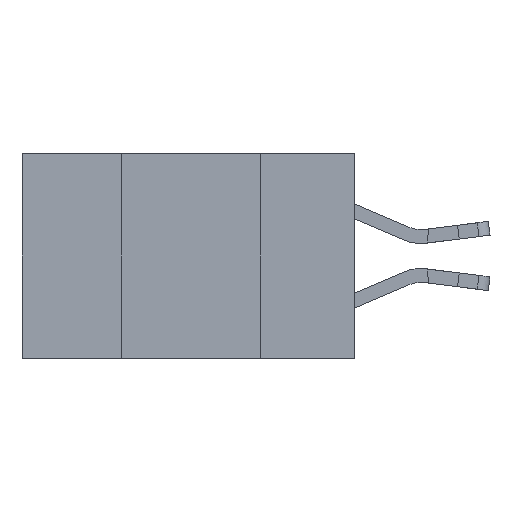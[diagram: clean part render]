
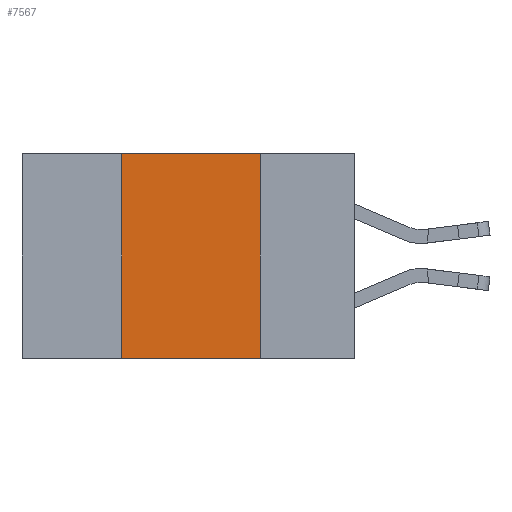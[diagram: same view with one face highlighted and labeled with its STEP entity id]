
A CAD part, left-side view. The second image highlights one B-rep face of the part: STEP entity #7567.
In plain terms, the highlighted planar face has unit normal (-1, 0, 0).
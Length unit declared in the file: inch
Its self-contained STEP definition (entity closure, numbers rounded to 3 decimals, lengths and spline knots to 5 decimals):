
#1269 = ORIENTED_EDGE ( 'NONE', *, *, #3879, .F. ) ;
#1408 = DIRECTION ( 'NONE',  ( 0., -1., 0. ) ) ;
#3184 = VERTEX_POINT ( 'NONE', #12324 ) ;
#3879 = EDGE_CURVE ( 'NONE', #6059, #7821, #13799, .T. ) ;
#4839 = EDGE_CURVE ( 'NONE', #8647, #3184, #12277, .T. ) ;
#4899 = DIRECTION ( 'NONE',  ( 0., 0., 1. ) ) ;
#4926 = CARTESIAN_POINT ( 'NONE',  ( 0., 0.42, 0. ) ) ;
#5412 = CARTESIAN_POINT ( 'NONE',  ( 0., 0.6, 0. ) ) ;
#5479 = ORIENTED_EDGE ( 'NONE', *, *, #13605, .F. ) ;
#5934 = AXIS2_PLACEMENT_3D ( 'NONE', #13303, #15640, #7866 ) ;
#6059 = VERTEX_POINT ( 'NONE', #10267 ) ;
#6491 = DIRECTION ( 'NONE',  ( 0., -1., 0. ) ) ;
#6593 = PLANE ( 'NONE',  #5934 ) ;
#6941 = ORIENTED_EDGE ( 'NONE', *, *, #4839, .F. ) ;
#7304 = CARTESIAN_POINT ( 'NONE',  ( 0., 0.42, -0.37 ) ) ;
#7508 = EDGE_LOOP ( 'NONE', ( #1269, #5479, #6941, #9437 ) ) ;
#7567 = ADVANCED_FACE ( 'NONE', ( #9948 ), #6593, .F. ) ;
#7821 = VERTEX_POINT ( 'NONE', #12943 ) ;
#7866 = DIRECTION ( 'NONE',  ( 0., 0., -1. ) ) ;
#8477 = DIRECTION ( 'NONE',  ( 0., 0., -1. ) ) ;
#8647 = VERTEX_POINT ( 'NONE', #7304 ) ;
#9334 = LINE ( 'NONE', #5412, #11555 ) ;
#9437 = ORIENTED_EDGE ( 'NONE', *, *, #10281, .T. ) ;
#9634 = LINE ( 'NONE', #14265, #16542 ) ;
#9948 = FACE_OUTER_BOUND ( 'NONE', #7508, .T. ) ;
#10267 = CARTESIAN_POINT ( 'NONE',  ( 0., 0.17, 0. ) ) ;
#10281 = EDGE_CURVE ( 'NONE', #8647, #7821, #9634, .T. ) ;
#10329 = VECTOR ( 'NONE', #8477, 39.37008 ) ;
#11555 = VECTOR ( 'NONE', #1408, 39.37008 ) ;
#12277 = LINE ( 'NONE', #4926, #15727 ) ;
#12324 = CARTESIAN_POINT ( 'NONE',  ( 0., 0.42, 0. ) ) ;
#12943 = CARTESIAN_POINT ( 'NONE',  ( 0., 0.17, -0.37 ) ) ;
#13303 = CARTESIAN_POINT ( 'NONE',  ( 0., 0.6, 0. ) ) ;
#13605 = EDGE_CURVE ( 'NONE', #3184, #6059, #9334, .T. ) ;
#13799 = LINE ( 'NONE', #15879, #10329 ) ;
#14265 = CARTESIAN_POINT ( 'NONE',  ( 0., 0.6, -0.37 ) ) ;
#15640 = DIRECTION ( 'NONE',  ( 1., 0., 0. ) ) ;
#15727 = VECTOR ( 'NONE', #4899, 39.37008 ) ;
#15879 = CARTESIAN_POINT ( 'NONE',  ( 0., 0.17, 0. ) ) ;
#16542 = VECTOR ( 'NONE', #6491, 39.37008 ) ;
